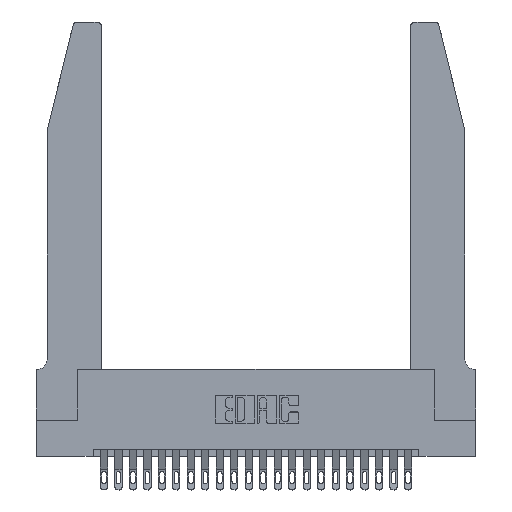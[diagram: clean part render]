
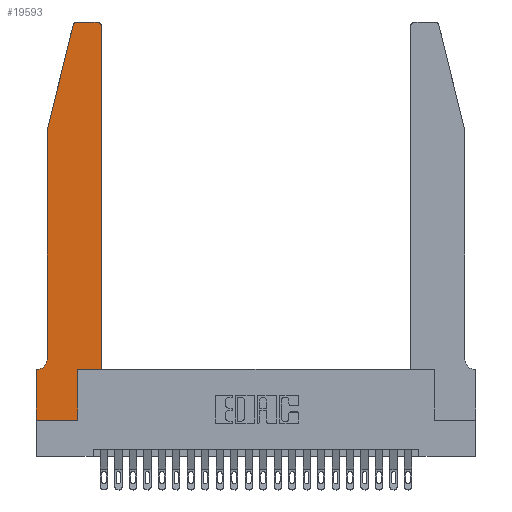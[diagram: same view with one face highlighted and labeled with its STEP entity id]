
A CAD part, top view. The second image highlights one B-rep face of the part: STEP entity #19593.
In plain terms, the highlighted planar face has unit normal (0, 0, 1).
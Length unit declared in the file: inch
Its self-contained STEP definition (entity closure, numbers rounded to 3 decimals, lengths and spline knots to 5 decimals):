
#505 = CARTESIAN_POINT ( 'NONE',  ( 0.284, 2.75, 0.37 ) ) ;
#513 = VERTEX_POINT ( 'NONE', #2564 ) ;
#682 = ORIENTED_EDGE ( 'NONE', *, *, #17194, .T. ) ;
#763 = CARTESIAN_POINT ( 'NONE',  ( 0.0755, 2., 0.37 ) ) ;
#873 = VECTOR ( 'NONE', #3177, 39.37008 ) ;
#1015 = CARTESIAN_POINT ( 'NONE',  ( 0.25487, 2.72718, 0.37 ) ) ;
#1030 = EDGE_CURVE ( 'NONE', #10299, #13823, #6904, .T. ) ;
#1168 = LINE ( 'NONE', #4837, #873 ) ;
#1549 = DIRECTION ( 'NONE',  ( -1., 0., 0. ) ) ;
#1836 = CARTESIAN_POINT ( 'NONE',  ( 0., 0., 0.37 ) ) ;
#2176 = CARTESIAN_POINT ( 'NONE',  ( 0.4205, 2.72, 0.37 ) ) ;
#2427 = CARTESIAN_POINT ( 'NONE',  ( 0.0755, 0.42, 0.37 ) ) ;
#2564 = CARTESIAN_POINT ( 'NONE',  ( 0., 0., 0.37 ) ) ;
#2852 = VECTOR ( 'NONE', #12512, 39.37008 ) ;
#3177 = DIRECTION ( 'NONE',  ( -0.239, -0.971, 0. ) ) ;
#3180 = DIRECTION ( 'NONE',  ( 1., 0., 0. ) ) ;
#3652 = VECTOR ( 'NONE', #15759, 39.37008 ) ;
#3777 = LINE ( 'NONE', #14318, #2852 ) ;
#3945 = DIRECTION ( 'NONE',  ( 0., 0., 1. ) ) ;
#4711 = DIRECTION ( 'NONE',  ( 0., 0., -1. ) ) ;
#4714 = VECTOR ( 'NONE', #23494, 39.37008 ) ;
#4772 = VERTEX_POINT ( 'NONE', #11899 ) ;
#4837 = CARTESIAN_POINT ( 'NONE',  ( 0.0755, 2., 0.37 ) ) ;
#5344 = ORIENTED_EDGE ( 'NONE', *, *, #23497, .T. ) ;
#5780 = VERTEX_POINT ( 'NONE', #1015 ) ;
#6067 = CARTESIAN_POINT ( 'NONE',  ( 0., 0.35, 0.37 ) ) ;
#6664 = AXIS2_PLACEMENT_3D ( 'NONE', #12778, #14752, #3180 ) ;
#6881 = CARTESIAN_POINT ( 'NONE',  ( 0.0055, 0.35, 0.37 ) ) ;
#6904 = LINE ( 'NONE', #21586, #11117 ) ;
#6988 = EDGE_CURVE ( 'NONE', #17543, #24116, #7513, .T. ) ;
#7513 = LINE ( 'NONE', #16895, #12618 ) ;
#7906 = EDGE_LOOP ( 'NONE', ( #23701, #8448, #24463, #20485, #5344, #7969, #23680, #11020, #21085, #22310, #21009, #682 ) ) ;
#7969 = ORIENTED_EDGE ( 'NONE', *, *, #6988, .T. ) ;
#8448 = ORIENTED_EDGE ( 'NONE', *, *, #23466, .T. ) ;
#8592 = EDGE_CURVE ( 'NONE', #10096, #11131, #10120, .T. ) ;
#8632 = CARTESIAN_POINT ( 'NONE',  ( 0.4505, 0.35, 0.37 ) ) ;
#9450 = VECTOR ( 'NONE', #10546, 39.37008 ) ;
#9858 = CARTESIAN_POINT ( 'NONE',  ( 0.284, 2.72, 0.37 ) ) ;
#9956 = AXIS2_PLACEMENT_3D ( 'NONE', #9858, #10028, #23500 ) ;
#9973 = CARTESIAN_POINT ( 'NONE',  ( 0.4505, 0.35, 0.37 ) ) ;
#10028 = DIRECTION ( 'NONE',  ( 0., 0., 1. ) ) ;
#10096 = VERTEX_POINT ( 'NONE', #763 ) ;
#10120 = LINE ( 'NONE', #16217, #4714 ) ;
#10299 = VERTEX_POINT ( 'NONE', #24460 ) ;
#10506 = VECTOR ( 'NONE', #15906, 39.37008 ) ;
#10546 = DIRECTION ( 'NONE',  ( 1., 0., 0. ) ) ;
#11020 = ORIENTED_EDGE ( 'NONE', *, *, #23330, .T. ) ;
#11117 = VECTOR ( 'NONE', #21998, 39.37008 ) ;
#11131 = VERTEX_POINT ( 'NONE', #2427 ) ;
#11422 = DIRECTION ( 'NONE',  ( 1., 0., 0. ) ) ;
#11605 = EDGE_CURVE ( 'NONE', #13823, #4772, #21615, .T. ) ;
#11899 = CARTESIAN_POINT ( 'NONE',  ( 0.4505, 0.35, 0.37 ) ) ;
#11995 = CARTESIAN_POINT ( 'NONE',  ( 0.4205, 2.75, 0.37 ) ) ;
#12512 = DIRECTION ( 'NONE',  ( -1., 0., 0. ) ) ;
#12555 = AXIS2_PLACEMENT_3D ( 'NONE', #15974, #4711, #24079 ) ;
#12618 = VECTOR ( 'NONE', #1549, 39.37008 ) ;
#12693 = PLANE ( 'NONE',  #6664 ) ;
#12778 = CARTESIAN_POINT ( 'NONE',  ( 0., 0.35, 0.37 ) ) ;
#13221 = LINE ( 'NONE', #1836, #22650 ) ;
#13823 = VERTEX_POINT ( 'NONE', #17245 ) ;
#13870 = LINE ( 'NONE', #21965, #10506 ) ;
#13977 = VERTEX_POINT ( 'NONE', #505 ) ;
#14318 = CARTESIAN_POINT ( 'NONE',  ( 0.2605, 2.75, 0.37 ) ) ;
#14601 = AXIS2_PLACEMENT_3D ( 'NONE', #2176, #3945, #21494 ) ;
#14752 = DIRECTION ( 'NONE',  ( 0., 0., 1. ) ) ;
#14763 = CIRCLE ( 'NONE', #14601, 0.03 ) ;
#15029 = CIRCLE ( 'NONE', #12555, 0.07 ) ;
#15759 = DIRECTION ( 'NONE',  ( 0., 1., 0. ) ) ;
#15906 = DIRECTION ( 'NONE',  ( 0., -1., 0. ) ) ;
#15974 = CARTESIAN_POINT ( 'NONE',  ( 0.0055, 0.42, 0.37 ) ) ;
#16217 = CARTESIAN_POINT ( 'NONE',  ( 0.0755, 2., 0.37 ) ) ;
#16344 = EDGE_CURVE ( 'NONE', #4772, #18573, #22444, .T. ) ;
#16682 = VERTEX_POINT ( 'NONE', #11995 ) ;
#16701 = EDGE_CURVE ( 'NONE', #24116, #513, #13870, .T. ) ;
#16895 = CARTESIAN_POINT ( 'NONE',  ( 0.0755, 0.35, 0.37 ) ) ;
#17194 = EDGE_CURVE ( 'NONE', #18573, #16682, #14763, .T. ) ;
#17245 = CARTESIAN_POINT ( 'NONE',  ( 0.2865, 0.35, 0.37 ) ) ;
#17543 = VERTEX_POINT ( 'NONE', #6881 ) ;
#17620 = EDGE_CURVE ( 'NONE', #5780, #10096, #1168, .T. ) ;
#18573 = VERTEX_POINT ( 'NONE', #19504 ) ;
#19368 = EDGE_CURVE ( 'NONE', #16682, #13977, #3777, .T. ) ;
#19504 = CARTESIAN_POINT ( 'NONE',  ( 0.4505, 2.72, 0.37 ) ) ;
#19558 = FACE_OUTER_BOUND ( 'NONE', #7906, .T. ) ;
#19593 = ADVANCED_FACE ( 'NONE', ( #19558 ), #12693, .T. ) ;
#20485 = ORIENTED_EDGE ( 'NONE', *, *, #8592, .T. ) ;
#21009 = ORIENTED_EDGE ( 'NONE', *, *, #16344, .T. ) ;
#21085 = ORIENTED_EDGE ( 'NONE', *, *, #1030, .T. ) ;
#21494 = DIRECTION ( 'NONE',  ( 1., 0., 0. ) ) ;
#21586 = CARTESIAN_POINT ( 'NONE',  ( 0.2865, 0.35, 0.37 ) ) ;
#21615 = LINE ( 'NONE', #8632, #9450 ) ;
#21965 = CARTESIAN_POINT ( 'NONE',  ( 0., 0., 0.37 ) ) ;
#21998 = DIRECTION ( 'NONE',  ( 0., 1., 0. ) ) ;
#22310 = ORIENTED_EDGE ( 'NONE', *, *, #11605, .T. ) ;
#22444 = LINE ( 'NONE', #9973, #3652 ) ;
#22650 = VECTOR ( 'NONE', #11422, 39.37008 ) ;
#23330 = EDGE_CURVE ( 'NONE', #513, #10299, #13221, .T. ) ;
#23466 = EDGE_CURVE ( 'NONE', #13977, #5780, #24145, .T. ) ;
#23494 = DIRECTION ( 'NONE',  ( 0., -1., 0. ) ) ;
#23497 = EDGE_CURVE ( 'NONE', #11131, #17543, #15029, .T. ) ;
#23500 = DIRECTION ( 'NONE',  ( 1., 0., 0. ) ) ;
#23680 = ORIENTED_EDGE ( 'NONE', *, *, #16701, .T. ) ;
#23701 = ORIENTED_EDGE ( 'NONE', *, *, #19368, .T. ) ;
#24079 = DIRECTION ( 'NONE',  ( -1., 0., 0. ) ) ;
#24116 = VERTEX_POINT ( 'NONE', #6067 ) ;
#24145 = CIRCLE ( 'NONE', #9956, 0.03 ) ;
#24460 = CARTESIAN_POINT ( 'NONE',  ( 0.2865, 0., 0.37 ) ) ;
#24463 = ORIENTED_EDGE ( 'NONE', *, *, #17620, .T. ) ;
